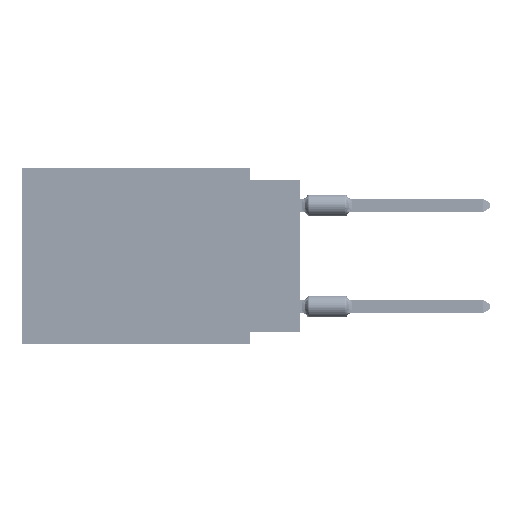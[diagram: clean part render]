
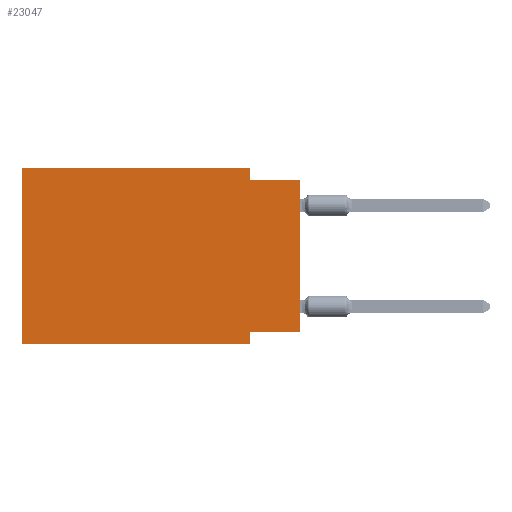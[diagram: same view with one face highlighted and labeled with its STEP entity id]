
A CAD part, left-side view. The second image highlights one B-rep face of the part: STEP entity #23047.
In plain terms, the highlighted planar face has unit normal (-1, 0, 0).
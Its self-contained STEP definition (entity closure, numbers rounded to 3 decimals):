
#997 = VERTEX_POINT ( 'NONE', #63458 ) ;
#1289 = DIRECTION ( 'NONE',  ( 0., 0., 1. ) ) ;
#2636 = DIRECTION ( 'NONE',  ( 1., 0., 0. ) ) ;
#2708 = CARTESIAN_POINT ( 'NONE',  ( 0., 13.97, 0. ) ) ;
#2736 = VECTOR ( 'NONE', #23093, 1000. ) ;
#3197 = CARTESIAN_POINT ( 'NONE',  ( 0., 0., 0. ) ) ;
#3393 = EDGE_CURVE ( 'NONE', #48471, #61081, #33961, .T. ) ;
#9240 = PLANE ( 'NONE',  #36172 ) ;
#11820 = EDGE_CURVE ( 'NONE', #41462, #997, #25464, .T. ) ;
#14787 = CARTESIAN_POINT ( 'NONE',  ( 0., 0., -0.635 ) ) ;
#17604 = VERTEX_POINT ( 'NONE', #2708 ) ;
#18850 = CARTESIAN_POINT ( 'NONE',  ( 0., 13.97, -8.89 ) ) ;
#19890 = ORIENTED_EDGE ( 'NONE', *, *, #63830, .F. ) ;
#22205 = EDGE_CURVE ( 'NONE', #60612, #38930, #66533, .T. ) ;
#22245 = CARTESIAN_POINT ( 'NONE',  ( 0., 13.97, 0. ) ) ;
#23047 = ADVANCED_FACE ( 'NONE', ( #29179 ), #9240, .F. ) ;
#23093 = DIRECTION ( 'NONE',  ( 0., 0., -1. ) ) ;
#23117 = LINE ( 'NONE', #49350, #26223 ) ;
#23615 = EDGE_CURVE ( 'NONE', #41051, #997, #48648, .T. ) ;
#23828 = VECTOR ( 'NONE', #35560, 1000. ) ;
#25464 = LINE ( 'NONE', #18850, #33652 ) ;
#26223 = VECTOR ( 'NONE', #55305, 1000. ) ;
#27207 = ORIENTED_EDGE ( 'NONE', *, *, #46823, .F. ) ;
#28254 = ORIENTED_EDGE ( 'NONE', *, *, #3393, .F. ) ;
#29179 = FACE_OUTER_BOUND ( 'NONE', #37576, .T. ) ;
#30552 = CARTESIAN_POINT ( 'NONE',  ( 0., 13.97, 0. ) ) ;
#31414 = CARTESIAN_POINT ( 'NONE',  ( 0., 13.97, -8.89 ) ) ;
#32069 = EDGE_CURVE ( 'NONE', #41462, #17604, #49167, .T. ) ;
#33652 = VECTOR ( 'NONE', #68143, 1000. ) ;
#33961 = LINE ( 'NONE', #60552, #59622 ) ;
#35560 = DIRECTION ( 'NONE',  ( 0., 1., 0. ) ) ;
#36172 = AXIS2_PLACEMENT_3D ( 'NONE', #30552, #2636, #40020 ) ;
#37576 = EDGE_LOOP ( 'NONE', ( #64170, #27207, #28254, #19890, #41926, #50344, #38475, #52132 ) ) ;
#38475 = ORIENTED_EDGE ( 'NONE', *, *, #23615, .F. ) ;
#38930 = VERTEX_POINT ( 'NONE', #14787 ) ;
#39242 = CARTESIAN_POINT ( 'NONE',  ( 0., 0., -8.255 ) ) ;
#39796 = LINE ( 'NONE', #60801, #23828 ) ;
#40020 = DIRECTION ( 'NONE',  ( 0., 0., -1. ) ) ;
#41051 = VERTEX_POINT ( 'NONE', #51210 ) ;
#41462 = VERTEX_POINT ( 'NONE', #31414 ) ;
#41926 = ORIENTED_EDGE ( 'NONE', *, *, #32069, .F. ) ;
#43307 = LINE ( 'NONE', #64645, #51717 ) ;
#44709 = CARTESIAN_POINT ( 'NONE',  ( 0., 2.54, 0. ) ) ;
#45063 = VECTOR ( 'NONE', #61271, 1000. ) ;
#45671 = EDGE_CURVE ( 'NONE', #60612, #41051, #39796, .T. ) ;
#46823 = EDGE_CURVE ( 'NONE', #61081, #38930, #23117, .T. ) ;
#48471 = VERTEX_POINT ( 'NONE', #44709 ) ;
#48569 = DIRECTION ( 'NONE',  ( 0., -1., 0. ) ) ;
#48648 = LINE ( 'NONE', #65085, #2736 ) ;
#49167 = LINE ( 'NONE', #22245, #54786 ) ;
#49350 = CARTESIAN_POINT ( 'NONE',  ( 0., 0., -0.635 ) ) ;
#50330 = CARTESIAN_POINT ( 'NONE',  ( 0., 2.54, -0.635 ) ) ;
#50344 = ORIENTED_EDGE ( 'NONE', *, *, #11820, .T. ) ;
#51210 = CARTESIAN_POINT ( 'NONE',  ( 0., 2.54, -8.255 ) ) ;
#51717 = VECTOR ( 'NONE', #48569, 1000. ) ;
#52132 = ORIENTED_EDGE ( 'NONE', *, *, #45671, .F. ) ;
#54786 = VECTOR ( 'NONE', #1289, 1000. ) ;
#55305 = DIRECTION ( 'NONE',  ( 0., -1., 0. ) ) ;
#59622 = VECTOR ( 'NONE', #66495, 1000. ) ;
#60552 = CARTESIAN_POINT ( 'NONE',  ( 0., 2.54, 0. ) ) ;
#60612 = VERTEX_POINT ( 'NONE', #39242 ) ;
#60801 = CARTESIAN_POINT ( 'NONE',  ( 0., 0., -8.255 ) ) ;
#61081 = VERTEX_POINT ( 'NONE', #50330 ) ;
#61271 = DIRECTION ( 'NONE',  ( 0., 0., 1. ) ) ;
#63458 = CARTESIAN_POINT ( 'NONE',  ( 0., 2.54, -8.89 ) ) ;
#63830 = EDGE_CURVE ( 'NONE', #17604, #48471, #43307, .T. ) ;
#64170 = ORIENTED_EDGE ( 'NONE', *, *, #22205, .T. ) ;
#64645 = CARTESIAN_POINT ( 'NONE',  ( 0., 13.97, 0. ) ) ;
#65085 = CARTESIAN_POINT ( 'NONE',  ( 0., 2.54, -8.89 ) ) ;
#66495 = DIRECTION ( 'NONE',  ( 0., 0., -1. ) ) ;
#66533 = LINE ( 'NONE', #3197, #45063 ) ;
#68143 = DIRECTION ( 'NONE',  ( 0., -1., 0. ) ) ;
